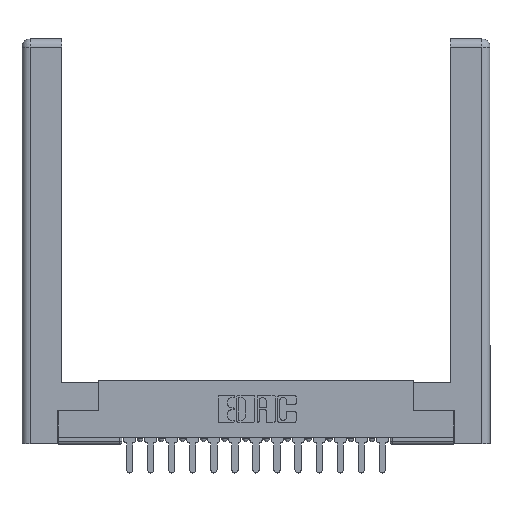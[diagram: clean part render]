
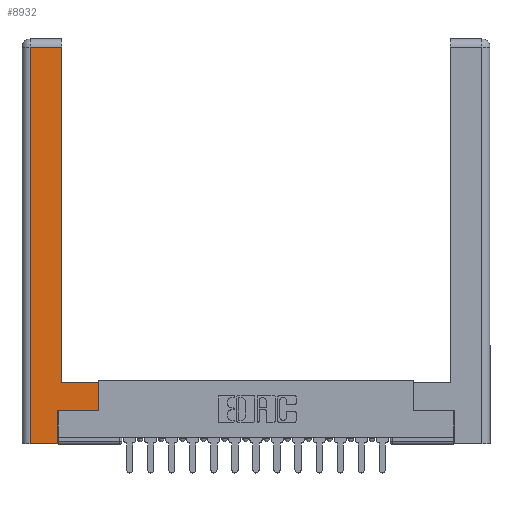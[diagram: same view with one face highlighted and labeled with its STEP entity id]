
A CAD part, top view. The second image highlights one B-rep face of the part: STEP entity #8932.
In plain terms, the highlighted planar face has unit normal (0, 0, 1).
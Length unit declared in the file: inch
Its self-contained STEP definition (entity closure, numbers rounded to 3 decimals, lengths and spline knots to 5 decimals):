
#366 = ORIENTED_EDGE ( 'NONE', *, *, #1141, .T. ) ;
#729 = ORIENTED_EDGE ( 'NONE', *, *, #2314, .T. ) ;
#894 = CARTESIAN_POINT ( 'NONE',  ( 0.0615, 2.94, 0. ) ) ;
#1141 = EDGE_CURVE ( 'NONE', #6840, #8984, #2033, .T. ) ;
#1856 = ORIENTED_EDGE ( 'NONE', *, *, #10756, .T. ) ;
#1892 = CARTESIAN_POINT ( 'NONE',  ( 0.295, 2.94, 0. ) ) ;
#1986 = ORIENTED_EDGE ( 'NONE', *, *, #14667, .T. ) ;
#2033 = LINE ( 'NONE', #15652, #2248 ) ;
#2104 = CARTESIAN_POINT ( 'NONE',  ( 0.295, 0.45, 0. ) ) ;
#2248 = VECTOR ( 'NONE', #10144, 39.37008 ) ;
#2314 = EDGE_CURVE ( 'NONE', #12551, #10424, #12274, .T. ) ;
#2398 = DIRECTION ( 'NONE',  ( -1., 0., 0. ) ) ;
#2475 = ORIENTED_EDGE ( 'NONE', *, *, #17333, .T. ) ;
#2818 = CARTESIAN_POINT ( 'NONE',  ( 0.265, 0.245, 0. ) ) ;
#3023 = CARTESIAN_POINT ( 'NONE',  ( 0.265, 0.245, 0. ) ) ;
#3609 = CARTESIAN_POINT ( 'NONE',  ( 0.295, 0.45, 0. ) ) ;
#4011 = VECTOR ( 'NONE', #8340, 39.37008 ) ;
#4497 = DIRECTION ( 'NONE',  ( 0., 1., 0. ) ) ;
#4782 = ORIENTED_EDGE ( 'NONE', *, *, #12487, .T. ) ;
#6780 = VECTOR ( 'NONE', #15040, 39.37008 ) ;
#6840 = VERTEX_POINT ( 'NONE', #1892 ) ;
#6979 = CARTESIAN_POINT ( 'NONE',  ( 0.265, 0., 0. ) ) ;
#7000 = LINE ( 'NONE', #10896, #15546 ) ;
#7083 = CARTESIAN_POINT ( 'NONE',  ( 0.0615, 0., 0. ) ) ;
#7705 = LINE ( 'NONE', #17261, #9558 ) ;
#7711 = DIRECTION ( 'NONE',  ( 1., 0., 0. ) ) ;
#8125 = CARTESIAN_POINT ( 'NONE',  ( 0.265, 0., 0. ) ) ;
#8197 = CARTESIAN_POINT ( 'NONE',  ( 0.565, 0.245, 0. ) ) ;
#8340 = DIRECTION ( 'NONE',  ( 1., 0., 0. ) ) ;
#8397 = CARTESIAN_POINT ( 'NONE',  ( 0.565, 0.45, 0. ) ) ;
#8932 = ADVANCED_FACE ( 'NONE', ( #15747 ), #17031, .F. ) ;
#8984 = VERTEX_POINT ( 'NONE', #894 ) ;
#9016 = DIRECTION ( 'NONE',  ( 0., 0., -1. ) ) ;
#9049 = LINE ( 'NONE', #2818, #6780 ) ;
#9143 = VERTEX_POINT ( 'NONE', #3023 ) ;
#9155 = VERTEX_POINT ( 'NONE', #6979 ) ;
#9441 = AXIS2_PLACEMENT_3D ( 'NONE', #14284, #9016, #11595 ) ;
#9513 = EDGE_CURVE ( 'NONE', #9155, #9143, #9049, .T. ) ;
#9558 = VECTOR ( 'NONE', #7711, 39.37008 ) ;
#10101 = VERTEX_POINT ( 'NONE', #8197 ) ;
#10144 = DIRECTION ( 'NONE',  ( -1., 0., 0. ) ) ;
#10424 = VERTEX_POINT ( 'NONE', #3609 ) ;
#10634 = ORIENTED_EDGE ( 'NONE', *, *, #9513, .T. ) ;
#10756 = EDGE_CURVE ( 'NONE', #8984, #10920, #7000, .T. ) ;
#10896 = CARTESIAN_POINT ( 'NONE',  ( 0.0615, 0., 0. ) ) ;
#10920 = VERTEX_POINT ( 'NONE', #7083 ) ;
#11016 = EDGE_LOOP ( 'NONE', ( #14011, #366, #1856, #4782, #10634, #1986, #2475, #729 ) ) ;
#11595 = DIRECTION ( 'NONE',  ( -1., 0., 0. ) ) ;
#12274 = LINE ( 'NONE', #2104, #14992 ) ;
#12487 = EDGE_CURVE ( 'NONE', #10920, #9155, #15513, .T. ) ;
#12551 = VERTEX_POINT ( 'NONE', #8397 ) ;
#13512 = LINE ( 'NONE', #13779, #13710 ) ;
#13710 = VECTOR ( 'NONE', #4497, 39.37008 ) ;
#13779 = CARTESIAN_POINT ( 'NONE',  ( 0.295, 3., 0. ) ) ;
#14011 = ORIENTED_EDGE ( 'NONE', *, *, #15610, .T. ) ;
#14284 = CARTESIAN_POINT ( 'NONE',  ( 0., 0., 0. ) ) ;
#14667 = EDGE_CURVE ( 'NONE', #9143, #10101, #7705, .T. ) ;
#14958 = DIRECTION ( 'NONE',  ( 0., -1., 0. ) ) ;
#14992 = VECTOR ( 'NONE', #2398, 39.37008 ) ;
#15040 = DIRECTION ( 'NONE',  ( 0., 1., 0. ) ) ;
#15370 = CARTESIAN_POINT ( 'NONE',  ( 0.565, 0.45, 0. ) ) ;
#15513 = LINE ( 'NONE', #8125, #4011 ) ;
#15546 = VECTOR ( 'NONE', #14958, 39.37008 ) ;
#15610 = EDGE_CURVE ( 'NONE', #10424, #6840, #13512, .T. ) ;
#15652 = CARTESIAN_POINT ( 'NONE',  ( 0.0615, 2.94, 0. ) ) ;
#15747 = FACE_OUTER_BOUND ( 'NONE', #11016, .T. ) ;
#16035 = VECTOR ( 'NONE', #16706, 39.37008 ) ;
#16456 = LINE ( 'NONE', #15370, #16035 ) ;
#16706 = DIRECTION ( 'NONE',  ( 0., 1., 0. ) ) ;
#17031 = PLANE ( 'NONE',  #9441 ) ;
#17261 = CARTESIAN_POINT ( 'NONE',  ( 0.565, 0.245, 0. ) ) ;
#17333 = EDGE_CURVE ( 'NONE', #10101, #12551, #16456, .T. ) ;
